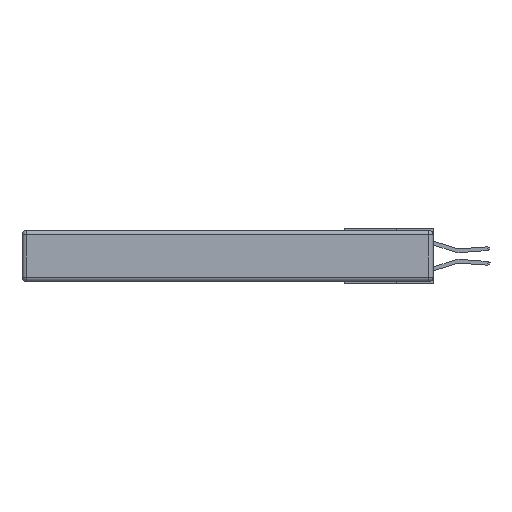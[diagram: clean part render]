
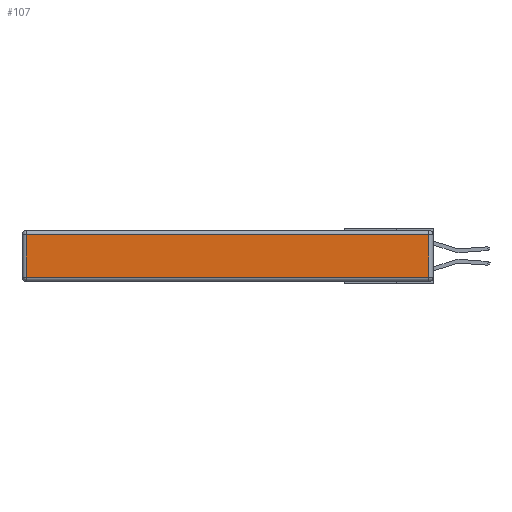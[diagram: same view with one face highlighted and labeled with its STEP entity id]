
A CAD part, left-side view. The second image highlights one B-rep face of the part: STEP entity #107.
In plain terms, the highlighted planar face has unit normal (-1, 0, 0).
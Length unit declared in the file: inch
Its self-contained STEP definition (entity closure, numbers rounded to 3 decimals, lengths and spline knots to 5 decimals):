
#107 = ADVANCED_FACE ( 'NONE', ( #292 ), #22579, .T. ) ;
#292 = FACE_OUTER_BOUND ( 'NONE', #5592, .T. ) ;
#1839 = DIRECTION ( 'NONE',  ( 0., 0., 1. ) ) ;
#2150 = LINE ( 'NONE', #12119, #5674 ) ;
#4145 = ORIENTED_EDGE ( 'NONE', *, *, #10458, .T. ) ;
#4311 = VERTEX_POINT ( 'NONE', #14000 ) ;
#4874 = DIRECTION ( 'NONE',  ( 0., 0., 1. ) ) ;
#5310 = DIRECTION ( 'NONE',  ( 0., 0., -1. ) ) ;
#5592 = EDGE_LOOP ( 'NONE', ( #17741, #15384, #8019, #4145 ) ) ;
#5674 = VECTOR ( 'NONE', #5310, 39.37008 ) ;
#6640 = CARTESIAN_POINT ( 'NONE',  ( 0., 0., -0.313 ) ) ;
#8019 = ORIENTED_EDGE ( 'NONE', *, *, #12603, .T. ) ;
#10374 = VECTOR ( 'NONE', #13371, 39.37008 ) ;
#10458 = EDGE_CURVE ( 'NONE', #19633, #4311, #2150, .T. ) ;
#10619 = EDGE_CURVE ( 'NONE', #23060, #26009, #15408, .T. ) ;
#12119 = CARTESIAN_POINT ( 'NONE',  ( 0., 2.72, -0.343 ) ) ;
#12510 = DIRECTION ( 'NONE',  ( 0., 1., 0. ) ) ;
#12603 = EDGE_CURVE ( 'NONE', #26009, #19633, #27612, .T. ) ;
#13371 = DIRECTION ( 'NONE',  ( 0., -1., 0. ) ) ;
#14000 = CARTESIAN_POINT ( 'NONE',  ( 0., 2.72, -0.313 ) ) ;
#14142 = EDGE_CURVE ( 'NONE', #4311, #23060, #27137, .T. ) ;
#15384 = ORIENTED_EDGE ( 'NONE', *, *, #10619, .T. ) ;
#15408 = LINE ( 'NONE', #28454, #20674 ) ;
#15867 = CARTESIAN_POINT ( 'NONE',  ( 0., 0., -0.343 ) ) ;
#16949 = CARTESIAN_POINT ( 'NONE',  ( 0., 0.03, -0.313 ) ) ;
#17741 = ORIENTED_EDGE ( 'NONE', *, *, #14142, .T. ) ;
#19633 = VERTEX_POINT ( 'NONE', #24875 ) ;
#20674 = VECTOR ( 'NONE', #1839, 39.37008 ) ;
#21429 = CARTESIAN_POINT ( 'NONE',  ( 0., 2.75, -0.03 ) ) ;
#22579 = PLANE ( 'NONE',  #27894 ) ;
#23060 = VERTEX_POINT ( 'NONE', #16949 ) ;
#24513 = DIRECTION ( 'NONE',  ( -1., 0., 0. ) ) ;
#24875 = CARTESIAN_POINT ( 'NONE',  ( 0., 2.72, -0.03 ) ) ;
#25125 = VECTOR ( 'NONE', #12510, 39.37008 ) ;
#26009 = VERTEX_POINT ( 'NONE', #26957 ) ;
#26957 = CARTESIAN_POINT ( 'NONE',  ( 0., 0.03, -0.03 ) ) ;
#27137 = LINE ( 'NONE', #6640, #10374 ) ;
#27612 = LINE ( 'NONE', #21429, #25125 ) ;
#27894 = AXIS2_PLACEMENT_3D ( 'NONE', #15867, #24513, #4874 ) ;
#28454 = CARTESIAN_POINT ( 'NONE',  ( 0., 0.03, -0.343 ) ) ;
